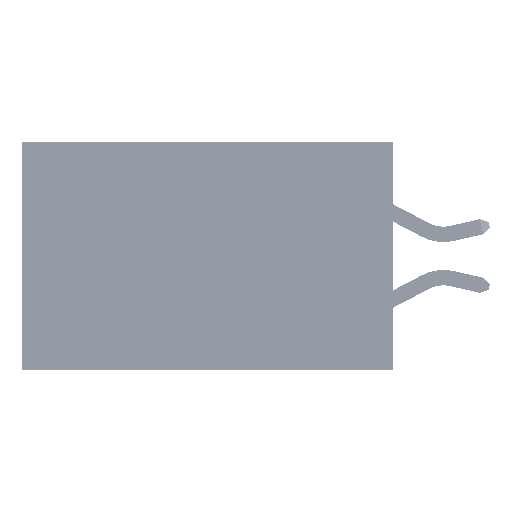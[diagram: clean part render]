
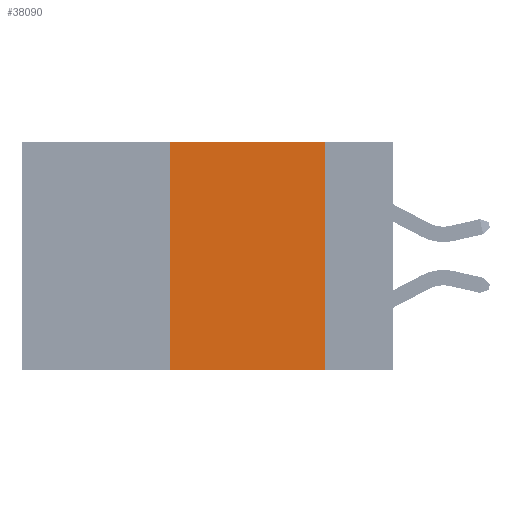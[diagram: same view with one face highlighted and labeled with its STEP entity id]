
A CAD part, left-side view. The second image highlights one B-rep face of the part: STEP entity #38090.
In plain terms, the highlighted planar face has unit normal (-1, 0, 0).
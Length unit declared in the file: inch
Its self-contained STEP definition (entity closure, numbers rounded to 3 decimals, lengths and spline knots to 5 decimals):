
#1435 = EDGE_CURVE ( 'NONE', #24718, #24226, #16951, .T. ) ;
#1597 = DIRECTION ( 'NONE',  ( 0., -1., 0. ) ) ;
#3850 = VECTOR ( 'NONE', #24769, 39.37008 ) ;
#4391 = CARTESIAN_POINT ( 'NONE',  ( 0., 0.36, 0. ) ) ;
#4477 = EDGE_LOOP ( 'NONE', ( #34923, #23244, #33363, #18947 ) ) ;
#8045 = CARTESIAN_POINT ( 'NONE',  ( 0., 0.6, 0. ) ) ;
#9481 = VERTEX_POINT ( 'NONE', #29785 ) ;
#11727 = LINE ( 'NONE', #39791, #36713 ) ;
#14704 = FACE_OUTER_BOUND ( 'NONE', #4477, .T. ) ;
#16951 = LINE ( 'NONE', #31651, #3850 ) ;
#18619 = DIRECTION ( 'NONE',  ( 0., 0., -1. ) ) ;
#18647 = LINE ( 'NONE', #19555, #37257 ) ;
#18947 = ORIENTED_EDGE ( 'NONE', *, *, #21614, .T. ) ;
#19055 = EDGE_CURVE ( 'NONE', #24226, #9481, #30956, .T. ) ;
#19555 = CARTESIAN_POINT ( 'NONE',  ( 0., 0.36, 0. ) ) ;
#19869 = EDGE_CURVE ( 'NONE', #44540, #24718, #18647, .T. ) ;
#21614 = EDGE_CURVE ( 'NONE', #44540, #9481, #11727, .T. ) ;
#22070 = PLANE ( 'NONE',  #27118 ) ;
#23244 = ORIENTED_EDGE ( 'NONE', *, *, #1435, .F. ) ;
#23407 = CARTESIAN_POINT ( 'NONE',  ( 0., 0.11, 0. ) ) ;
#24226 = VERTEX_POINT ( 'NONE', #29269 ) ;
#24718 = VERTEX_POINT ( 'NONE', #4391 ) ;
#24755 = VECTOR ( 'NONE', #41571, 39.37008 ) ;
#24769 = DIRECTION ( 'NONE',  ( 0., -1., 0. ) ) ;
#27118 = AXIS2_PLACEMENT_3D ( 'NONE', #8045, #43698, #18619 ) ;
#29269 = CARTESIAN_POINT ( 'NONE',  ( 0., 0.11, 0. ) ) ;
#29785 = CARTESIAN_POINT ( 'NONE',  ( 0., 0.11, -0.37 ) ) ;
#30956 = LINE ( 'NONE', #23407, #24755 ) ;
#31651 = CARTESIAN_POINT ( 'NONE',  ( 0., 0.6, 0. ) ) ;
#33363 = ORIENTED_EDGE ( 'NONE', *, *, #19869, .F. ) ;
#33567 = DIRECTION ( 'NONE',  ( 0., 0., 1. ) ) ;
#34923 = ORIENTED_EDGE ( 'NONE', *, *, #19055, .F. ) ;
#36713 = VECTOR ( 'NONE', #1597, 39.37008 ) ;
#37257 = VECTOR ( 'NONE', #33567, 39.37008 ) ;
#38090 = ADVANCED_FACE ( 'NONE', ( #14704 ), #22070, .F. ) ;
#39791 = CARTESIAN_POINT ( 'NONE',  ( 0., 0.6, -0.37 ) ) ;
#39856 = CARTESIAN_POINT ( 'NONE',  ( 0., 0.36, -0.37 ) ) ;
#41571 = DIRECTION ( 'NONE',  ( 0., 0., -1. ) ) ;
#43698 = DIRECTION ( 'NONE',  ( 1., 0., 0. ) ) ;
#44540 = VERTEX_POINT ( 'NONE', #39856 ) ;
